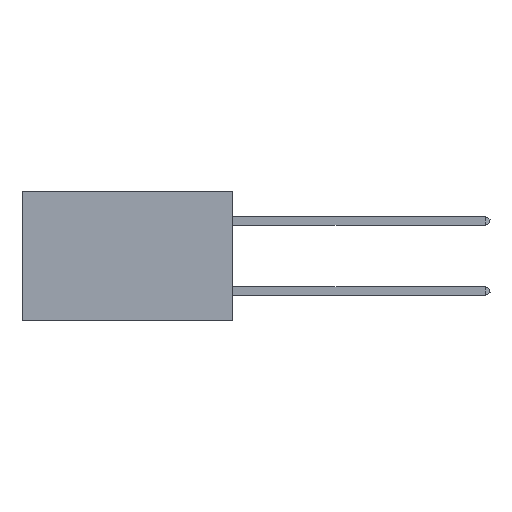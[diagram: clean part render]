
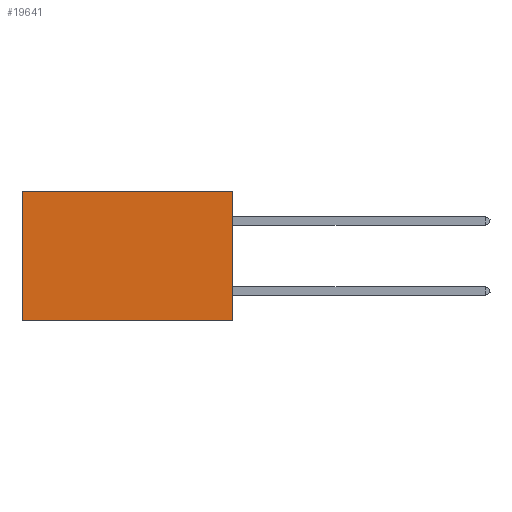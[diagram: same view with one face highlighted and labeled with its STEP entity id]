
A CAD part, left-side view. The second image highlights one B-rep face of the part: STEP entity #19641.
In plain terms, the highlighted planar face has unit normal (-1, 0, 0).
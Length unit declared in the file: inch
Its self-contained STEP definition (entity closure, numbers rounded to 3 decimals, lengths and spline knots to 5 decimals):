
#241 = DIRECTION ( 'NONE',  ( 0., 0., -1. ) ) ;
#6113 = EDGE_CURVE ( 'NONE', #39099, #24650, #37756, .T. ) ;
#11265 = ORIENTED_EDGE ( 'NONE', *, *, #22959, .F. ) ;
#12445 = VECTOR ( 'NONE', #30588, 39.37008 ) ;
#13942 = EDGE_CURVE ( 'NONE', #39099, #37065, #18824, .T. ) ;
#14150 = DIRECTION ( 'NONE',  ( 0., 1., 0. ) ) ;
#14647 = EDGE_LOOP ( 'NONE', ( #15301, #11265, #43082, #16349 ) ) ;
#15301 = ORIENTED_EDGE ( 'NONE', *, *, #35990, .T. ) ;
#16349 = ORIENTED_EDGE ( 'NONE', *, *, #13942, .T. ) ;
#16359 = CARTESIAN_POINT ( 'NONE',  ( 0.2875, 0., 0. ) ) ;
#16593 = VECTOR ( 'NONE', #39424, 39.37008 ) ;
#17328 = CARTESIAN_POINT ( 'NONE',  ( 0.2875, 0., 0. ) ) ;
#17375 = CARTESIAN_POINT ( 'NONE',  ( 0.2875, 0., -0.37 ) ) ;
#18664 = CARTESIAN_POINT ( 'NONE',  ( 0.2875, 0.6, -0.37 ) ) ;
#18824 = LINE ( 'NONE', #20962, #24031 ) ;
#19608 = VECTOR ( 'NONE', #26637, 39.37008 ) ;
#19641 = ADVANCED_FACE ( 'NONE', ( #34756 ), #37767, .F. ) ;
#20752 = DIRECTION ( 'NONE',  ( 1., 0., 0. ) ) ;
#20962 = CARTESIAN_POINT ( 'NONE',  ( 0.2875, 0., 0. ) ) ;
#21455 = LINE ( 'NONE', #40705, #12445 ) ;
#22959 = EDGE_CURVE ( 'NONE', #24650, #39077, #42706, .T. ) ;
#23315 = AXIS2_PLACEMENT_3D ( 'NONE', #17328, #20752, #241 ) ;
#24031 = VECTOR ( 'NONE', #14150, 39.37008 ) ;
#24650 = VERTEX_POINT ( 'NONE', #17375 ) ;
#26637 = DIRECTION ( 'NONE',  ( 0., 0., -1. ) ) ;
#30588 = DIRECTION ( 'NONE',  ( 0., 0., -1. ) ) ;
#32579 = CARTESIAN_POINT ( 'NONE',  ( 0.2875, 0.6, 0. ) ) ;
#34756 = FACE_OUTER_BOUND ( 'NONE', #14647, .T. ) ;
#35679 = CARTESIAN_POINT ( 'NONE',  ( 0.2875, 0., 0. ) ) ;
#35990 = EDGE_CURVE ( 'NONE', #37065, #39077, #21455, .T. ) ;
#36022 = CARTESIAN_POINT ( 'NONE',  ( 0.2875, 0., -0.37 ) ) ;
#37065 = VERTEX_POINT ( 'NONE', #32579 ) ;
#37756 = LINE ( 'NONE', #16359, #19608 ) ;
#37767 = PLANE ( 'NONE',  #23315 ) ;
#39077 = VERTEX_POINT ( 'NONE', #18664 ) ;
#39099 = VERTEX_POINT ( 'NONE', #35679 ) ;
#39424 = DIRECTION ( 'NONE',  ( 0., 1., 0. ) ) ;
#40705 = CARTESIAN_POINT ( 'NONE',  ( 0.2875, 0.6, 0. ) ) ;
#42706 = LINE ( 'NONE', #36022, #16593 ) ;
#43082 = ORIENTED_EDGE ( 'NONE', *, *, #6113, .F. ) ;
